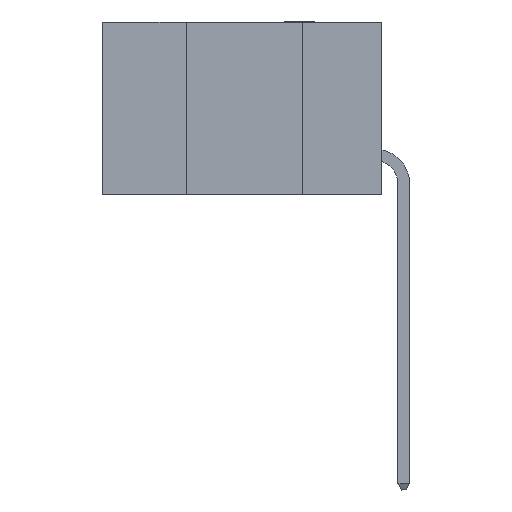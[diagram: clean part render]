
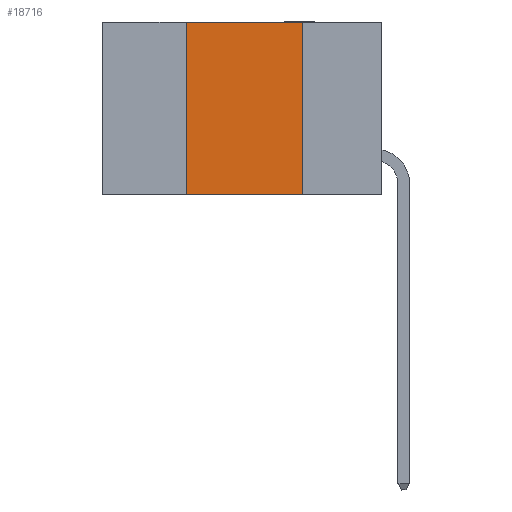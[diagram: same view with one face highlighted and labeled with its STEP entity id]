
A CAD part, left-side view. The second image highlights one B-rep face of the part: STEP entity #18716.
In plain terms, the highlighted planar face has unit normal (-1, 0, 0).
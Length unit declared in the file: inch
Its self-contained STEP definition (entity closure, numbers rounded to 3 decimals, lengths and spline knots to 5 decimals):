
#887 = LINE ( 'NONE', #14134, #11623 ) ;
#1011 = VECTOR ( 'NONE', #1283, 39.37008 ) ;
#1265 = DIRECTION ( 'NONE',  ( 0., -1., 0. ) ) ;
#1283 = DIRECTION ( 'NONE',  ( 0., -1., 0. ) ) ;
#1715 = CARTESIAN_POINT ( 'NONE',  ( 0., 0.17, -0.37 ) ) ;
#2216 = CARTESIAN_POINT ( 'NONE',  ( 0., 0.6, 0. ) ) ;
#2285 = LINE ( 'NONE', #8528, #17762 ) ;
#2826 = ORIENTED_EDGE ( 'NONE', *, *, #18329, .F. ) ;
#3481 = EDGE_CURVE ( 'NONE', #18429, #18650, #13164, .T. ) ;
#3614 = DIRECTION ( 'NONE',  ( 0., 0., -1. ) ) ;
#4081 = DIRECTION ( 'NONE',  ( 0., 0., -1. ) ) ;
#4764 = CARTESIAN_POINT ( 'NONE',  ( 0., 0.17, 0. ) ) ;
#4874 = FACE_OUTER_BOUND ( 'NONE', #7229, .T. ) ;
#5641 = VECTOR ( 'NONE', #4081, 39.37008 ) ;
#6624 = ORIENTED_EDGE ( 'NONE', *, *, #11952, .F. ) ;
#6885 = VERTEX_POINT ( 'NONE', #4764 ) ;
#7209 = CARTESIAN_POINT ( 'NONE',  ( 0., 0.17, 0. ) ) ;
#7229 = EDGE_LOOP ( 'NONE', ( #6624, #2826, #9954, #17112 ) ) ;
#7606 = CARTESIAN_POINT ( 'NONE',  ( 0., 0.42, -0.37 ) ) ;
#7998 = PLANE ( 'NONE',  #13041 ) ;
#8171 = DIRECTION ( 'NONE',  ( 0., 0., 1. ) ) ;
#8528 = CARTESIAN_POINT ( 'NONE',  ( 0., 0.6, 0. ) ) ;
#9954 = ORIENTED_EDGE ( 'NONE', *, *, #18731, .F. ) ;
#10371 = CARTESIAN_POINT ( 'NONE',  ( 0., 0.6, -0.37 ) ) ;
#11284 = CARTESIAN_POINT ( 'NONE',  ( 0., 0.42, 0. ) ) ;
#11623 = VECTOR ( 'NONE', #8171, 39.37008 ) ;
#11952 = EDGE_CURVE ( 'NONE', #6885, #18650, #13098, .T. ) ;
#13041 = AXIS2_PLACEMENT_3D ( 'NONE', #2216, #15656, #3614 ) ;
#13098 = LINE ( 'NONE', #7209, #5641 ) ;
#13164 = LINE ( 'NONE', #10371, #1011 ) ;
#14134 = CARTESIAN_POINT ( 'NONE',  ( 0., 0.42, 0. ) ) ;
#15656 = DIRECTION ( 'NONE',  ( 1., 0., 0. ) ) ;
#16372 = VERTEX_POINT ( 'NONE', #11284 ) ;
#17112 = ORIENTED_EDGE ( 'NONE', *, *, #3481, .T. ) ;
#17762 = VECTOR ( 'NONE', #1265, 39.37008 ) ;
#18329 = EDGE_CURVE ( 'NONE', #16372, #6885, #2285, .T. ) ;
#18429 = VERTEX_POINT ( 'NONE', #7606 ) ;
#18650 = VERTEX_POINT ( 'NONE', #1715 ) ;
#18716 = ADVANCED_FACE ( 'NONE', ( #4874 ), #7998, .F. ) ;
#18731 = EDGE_CURVE ( 'NONE', #18429, #16372, #887, .T. ) ;
